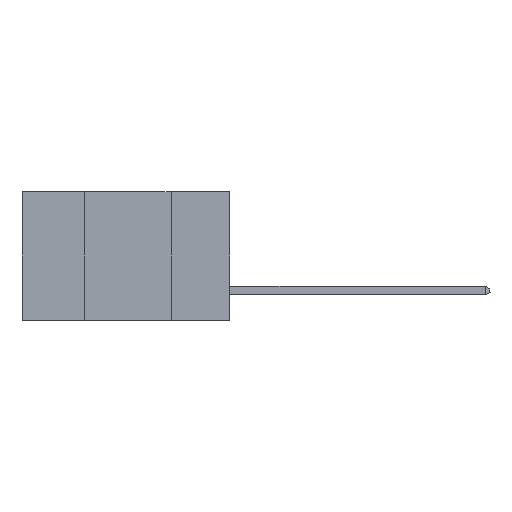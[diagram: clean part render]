
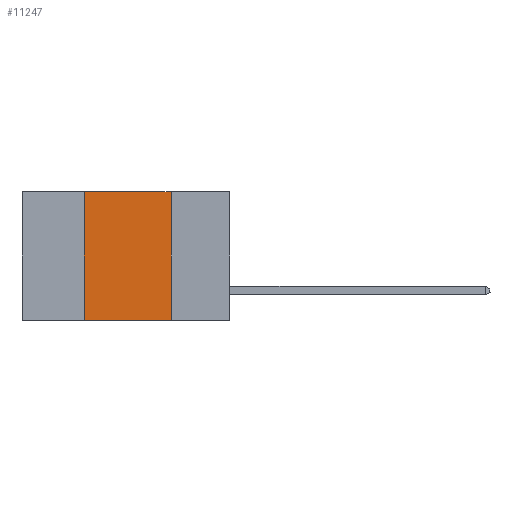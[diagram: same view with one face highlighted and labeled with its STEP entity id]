
A CAD part, left-side view. The second image highlights one B-rep face of the part: STEP entity #11247.
In plain terms, the highlighted planar face has unit normal (-1, 0, 0).
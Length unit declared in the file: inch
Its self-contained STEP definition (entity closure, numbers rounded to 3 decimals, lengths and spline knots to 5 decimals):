
#1202 = CARTESIAN_POINT ( 'NONE',  ( 0., 0.42, -0.37 ) ) ;
#1260 = VERTEX_POINT ( 'NONE', #3664 ) ;
#2904 = LINE ( 'NONE', #6290, #13113 ) ;
#3260 = DIRECTION ( 'NONE',  ( 0., 0., -1. ) ) ;
#3664 = CARTESIAN_POINT ( 'NONE',  ( 0., 0.42, 0. ) ) ;
#3728 = LINE ( 'NONE', #10209, #10581 ) ;
#4401 = ORIENTED_EDGE ( 'NONE', *, *, #10794, .T. ) ;
#4740 = CARTESIAN_POINT ( 'NONE',  ( 0., 0.6, 0. ) ) ;
#5088 = CARTESIAN_POINT ( 'NONE',  ( 0., 0.17, -0.37 ) ) ;
#5511 = ORIENTED_EDGE ( 'NONE', *, *, #8746, .F. ) ;
#6290 = CARTESIAN_POINT ( 'NONE',  ( 0., 0.6, -0.37 ) ) ;
#6364 = DIRECTION ( 'NONE',  ( 0., -1., 0. ) ) ;
#6788 = VECTOR ( 'NONE', #9471, 39.37008 ) ;
#7958 = PLANE ( 'NONE',  #15907 ) ;
#8245 = LINE ( 'NONE', #4740, #6788 ) ;
#8746 = EDGE_CURVE ( 'NONE', #1260, #19498, #8245, .T. ) ;
#8769 = FACE_OUTER_BOUND ( 'NONE', #11761, .T. ) ;
#9471 = DIRECTION ( 'NONE',  ( 0., -1., 0. ) ) ;
#9560 = DIRECTION ( 'NONE',  ( 1., 0., 0. ) ) ;
#10209 = CARTESIAN_POINT ( 'NONE',  ( 0., 0.17, 0. ) ) ;
#10581 = VECTOR ( 'NONE', #19587, 39.37008 ) ;
#10794 = EDGE_CURVE ( 'NONE', #17959, #15078, #2904, .T. ) ;
#11247 = ADVANCED_FACE ( 'NONE', ( #8769 ), #7958, .F. ) ;
#11761 = EDGE_LOOP ( 'NONE', ( #17368, #5511, #18562, #4401 ) ) ;
#11922 = CARTESIAN_POINT ( 'NONE',  ( 0., 0.17, 0. ) ) ;
#13040 = CARTESIAN_POINT ( 'NONE',  ( 0., 0.42, 0. ) ) ;
#13113 = VECTOR ( 'NONE', #6364, 39.37008 ) ;
#13190 = EDGE_CURVE ( 'NONE', #17959, #1260, #16189, .T. ) ;
#13532 = VECTOR ( 'NONE', #17971, 39.37008 ) ;
#15078 = VERTEX_POINT ( 'NONE', #5088 ) ;
#15424 = CARTESIAN_POINT ( 'NONE',  ( 0., 0.6, 0. ) ) ;
#15907 = AXIS2_PLACEMENT_3D ( 'NONE', #15424, #9560, #3260 ) ;
#16189 = LINE ( 'NONE', #13040, #13532 ) ;
#17345 = EDGE_CURVE ( 'NONE', #19498, #15078, #3728, .T. ) ;
#17368 = ORIENTED_EDGE ( 'NONE', *, *, #17345, .F. ) ;
#17959 = VERTEX_POINT ( 'NONE', #1202 ) ;
#17971 = DIRECTION ( 'NONE',  ( 0., 0., 1. ) ) ;
#18562 = ORIENTED_EDGE ( 'NONE', *, *, #13190, .F. ) ;
#19498 = VERTEX_POINT ( 'NONE', #11922 ) ;
#19587 = DIRECTION ( 'NONE',  ( 0., 0., -1. ) ) ;
